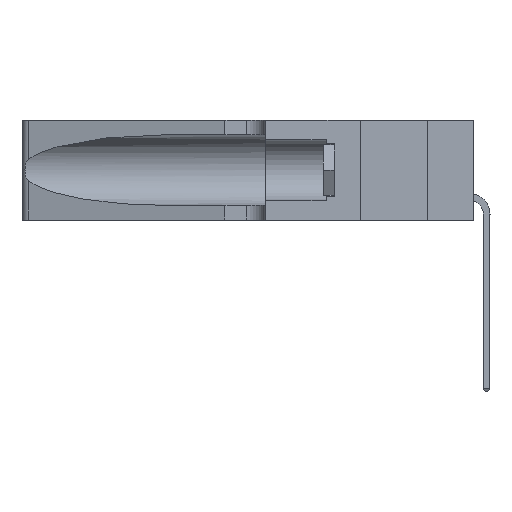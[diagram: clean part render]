
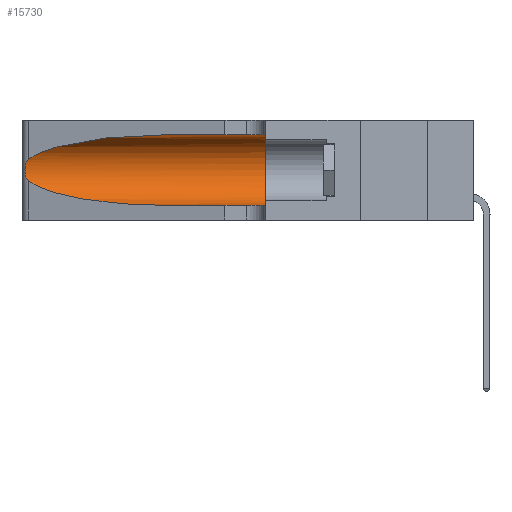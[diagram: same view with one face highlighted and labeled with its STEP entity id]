
A CAD part, left-side view. The second image highlights one B-rep face of the part: STEP entity #15730.
In plain terms, the highlighted cylindrical face has radius 3.308 mm (diameter 6.617 mm), a partial arc.
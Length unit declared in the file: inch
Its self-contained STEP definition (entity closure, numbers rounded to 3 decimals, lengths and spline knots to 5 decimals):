
#198 = AXIS2_PLACEMENT_3D ( 'NONE', #19545, #2434, #2594 ) ;
#395 = CYLINDRICAL_SURFACE ( 'NONE', #198, 0.13025 ) ;
#772 = VERTEX_POINT ( 'NONE', #1359 ) ;
#825 = CARTESIAN_POINT ( 'NONE',  ( 0.25854, 1.2359, 0.20912 ) ) ;
#1007 = VECTOR ( 'NONE', #9555, 39.37008 ) ;
#1129 = CARTESIAN_POINT ( 'NONE',  ( 0.25639, 1.23186, 0.15144 ) ) ;
#1359 = CARTESIAN_POINT ( 'NONE',  ( 0.25487, 1.22718, 0.14631 ) ) ;
#1724 = CARTESIAN_POINT ( 'NONE',  ( 0.25487, 1.22718, 0.14631 ) ) ;
#2168 = CARTESIAN_POINT ( 'NONE',  ( 0.1305, 0.72297, 0.05475 ) ) ;
#2390 = EDGE_CURVE ( 'NONE', #37734, #11690, #3715, .T. ) ;
#2434 = DIRECTION ( 'NONE',  ( 0., -1., 0. ) ) ;
#2594 = DIRECTION ( 'NONE',  ( 0., 0., -1. ) ) ;
#3715 = LINE ( 'NONE', #8046, #1007 ) ;
#3977 = CARTESIAN_POINT ( 'NONE',  ( 0.26017, 1.23833, 0.17102 ) ) ;
#4267 = ORIENTED_EDGE ( 'NONE', *, *, #2390, .F. ) ;
#6701 = CARTESIAN_POINT ( 'NONE',  ( 0.25639, 1.23184, 0.21858 ) ) ;
#7661 = ORIENTED_EDGE ( 'NONE', *, *, #22982, .T. ) ;
#8026 = CARTESIAN_POINT ( 'NONE',  ( 0.1305, 0.72297, 0.05475 ) ) ;
#8046 = CARTESIAN_POINT ( 'NONE',  ( 0.1305, 1.61858, 0.31525 ) ) ;
#8863 = EDGE_CURVE ( 'NONE', #28237, #31062, #30618, .T. ) ;
#9555 = DIRECTION ( 'NONE',  ( 0., -1., 0. ) ) ;
#9765 = CARTESIAN_POINT ( 'NONE',  ( 0.1305, 0.35, 0.185 ) ) ;
#10437 = ORIENTED_EDGE ( 'NONE', *, *, #30764, .F. ) ;
#10808 = CARTESIAN_POINT ( 'NONE',  ( 0.1305, 0.72297, 0.31525 ) ) ;
#10928 = FACE_OUTER_BOUND ( 'NONE', #13687, .T. ) ;
#11113 = CARTESIAN_POINT ( 'NONE',  ( 0.26075, 1.23896, 0.19203 ) ) ;
#11190 = CARTESIAN_POINT ( 'NONE',  ( 0.25487, 1.22718, 0.22369 ) ) ;
#11426 = CARTESIAN_POINT ( 'NONE',  ( 0.1305, 1.61858, 0.05475 ) ) ;
#11690 = VERTEX_POINT ( 'NONE', #18196 ) ;
#13513 = ORIENTED_EDGE ( 'NONE', *, *, #21335, .T. ) ;
#13687 = EDGE_LOOP ( 'NONE', ( #7661, #13513, #22555, #18795, #10437, #4267 ) ) ;
#14903 = B_SPLINE_CURVE_WITH_KNOTS ( 'NONE', 3,
 ( #33587, #26989, #6701, #40003, #825, #40685, #11113, #23910, #3977, #27545, #41140, #1129, #27838, #1724 ),
 .UNSPECIFIED., .F., .F.,
 ( 4, 2, 2, 2, 2, 2, 4 ),
 ( 0., 0.00027, 0.00053, 0.00107, 0.0016, 0.00187, 0.00214 ),
 .UNSPECIFIED. ) ;
#15730 = ADVANCED_FACE ( 'NONE', ( #10928 ), #395, .F. ) ;
#16448 = DIRECTION ( 'NONE',  ( 0., 0., 1. ) ) ;
#18128 = DIRECTION ( 'NONE',  ( 0., -1., 0. ) ) ;
#18196 = CARTESIAN_POINT ( 'NONE',  ( 0.1305, 0.35, 0.31525 ) ) ;
#18795 = ORIENTED_EDGE ( 'NONE', *, *, #8863, .T. ) ;
#18818 = CARTESIAN_POINT ( 'NONE',  ( 0.2373, 1.15595, 0.08982 ) ) ;
#19545 = CARTESIAN_POINT ( 'NONE',  ( 0.1305, 1.61858, 0.185 ) ) ;
#19902 = AXIS2_PLACEMENT_3D ( 'NONE', #9765, #33038, #16448 ) ;
#21335 = EDGE_CURVE ( 'NONE', #26273, #772, #14903, .T. ) ;
#22555 = ORIENTED_EDGE ( 'NONE', *, *, #30104, .T. ) ;
#22982 = EDGE_CURVE ( 'NONE', #37734, #26273, #25579, .T. ) ;
#23910 = CARTESIAN_POINT ( 'NONE',  ( 0.26075, 1.23896, 0.178 ) ) ;
#25579 =( BOUNDED_CURVE ( )  B_SPLINE_CURVE ( 3, ( #42469, #36609, #32809, #11190 ),
 .UNSPECIFIED., .F., .T. ) 
 B_SPLINE_CURVE_WITH_KNOTS ( ( 4, 4 ),
 ( 1.5708, 2.84003 ),
 .UNSPECIFIED. ) 
 CURVE ( )  GEOMETRIC_REPRESENTATION_ITEM ( )  RATIONAL_B_SPLINE_CURVE ( ( 1., 0.87, 0.87, 1. ) ) 
 REPRESENTATION_ITEM ( '' )  );
#26149 =( BOUNDED_CURVE ( )  B_SPLINE_CURVE ( 3, ( #28553, #18818, #42176, #2168 ),
 .UNSPECIFIED., .F., .T. ) 
 B_SPLINE_CURVE_WITH_KNOTS ( ( 4, 4 ),
 ( 3.44316, 4.71239 ),
 .UNSPECIFIED. ) 
 CURVE ( )  GEOMETRIC_REPRESENTATION_ITEM ( )  RATIONAL_B_SPLINE_CURVE ( ( 1., 0.87, 0.87, 1. ) ) 
 REPRESENTATION_ITEM ( '' )  );
#26273 = VERTEX_POINT ( 'NONE', #38328 ) ;
#26287 = CIRCLE ( 'NONE', #19902, 0.13025 ) ;
#26989 = CARTESIAN_POINT ( 'NONE',  ( 0.25555, 1.22994, 0.2215 ) ) ;
#27545 = CARTESIAN_POINT ( 'NONE',  ( 0.25856, 1.23593, 0.16098 ) ) ;
#27838 = CARTESIAN_POINT ( 'NONE',  ( 0.25555, 1.22993, 0.14849 ) ) ;
#28237 = VERTEX_POINT ( 'NONE', #8026 ) ;
#28553 = CARTESIAN_POINT ( 'NONE',  ( 0.25487, 1.22718, 0.14631 ) ) ;
#30104 = EDGE_CURVE ( 'NONE', #772, #28237, #26149, .T. ) ;
#30618 = LINE ( 'NONE', #11426, #34252 ) ;
#30764 = EDGE_CURVE ( 'NONE', #11690, #31062, #26287, .T. ) ;
#31062 = VERTEX_POINT ( 'NONE', #40706 ) ;
#32809 = CARTESIAN_POINT ( 'NONE',  ( 0.2373, 1.15595, 0.28018 ) ) ;
#33038 = DIRECTION ( 'NONE',  ( 0., 1., 0. ) ) ;
#33587 = CARTESIAN_POINT ( 'NONE',  ( 0.25487, 1.22718, 0.22369 ) ) ;
#34252 = VECTOR ( 'NONE', #18128, 39.37008 ) ;
#36609 = CARTESIAN_POINT ( 'NONE',  ( 0.18966, 0.96281, 0.31525 ) ) ;
#37734 = VERTEX_POINT ( 'NONE', #10808 ) ;
#38328 = CARTESIAN_POINT ( 'NONE',  ( 0.25487, 1.22718, 0.22369 ) ) ;
#40003 = CARTESIAN_POINT ( 'NONE',  ( 0.25787, 1.23484, 0.2124 ) ) ;
#40685 = CARTESIAN_POINT ( 'NONE',  ( 0.26018, 1.23835, 0.19895 ) ) ;
#40706 = CARTESIAN_POINT ( 'NONE',  ( 0.1305, 0.35, 0.05475 ) ) ;
#41140 = CARTESIAN_POINT ( 'NONE',  ( 0.25789, 1.23486, 0.15765 ) ) ;
#42176 = CARTESIAN_POINT ( 'NONE',  ( 0.18966, 0.96281, 0.05475 ) ) ;
#42469 = CARTESIAN_POINT ( 'NONE',  ( 0.1305, 0.72297, 0.31525 ) ) ;
